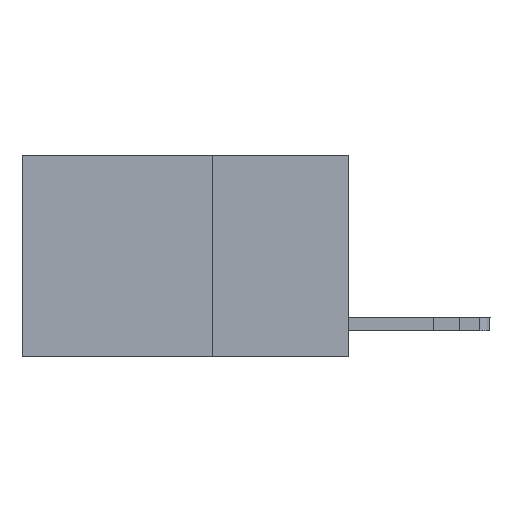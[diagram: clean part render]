
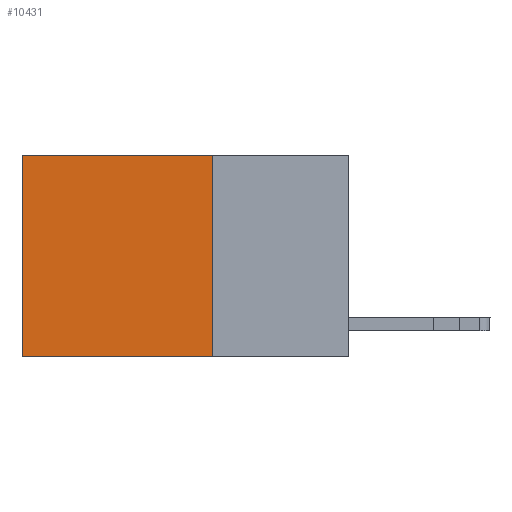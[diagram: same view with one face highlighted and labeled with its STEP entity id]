
A CAD part, left-side view. The second image highlights one B-rep face of the part: STEP entity #10431.
In plain terms, the highlighted planar face has unit normal (-1, 0, 0).
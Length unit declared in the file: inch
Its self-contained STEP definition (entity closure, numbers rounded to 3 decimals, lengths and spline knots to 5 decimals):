
#538 = PLANE ( 'NONE',  #15681 ) ;
#668 = VERTEX_POINT ( 'NONE', #9361 ) ;
#763 = ORIENTED_EDGE ( 'NONE', *, *, #8761, .F. ) ;
#1284 = EDGE_CURVE ( 'NONE', #5396, #668, #12461, .T. ) ;
#1404 = CARTESIAN_POINT ( 'NONE',  ( 0.2625, 0.6, -0.37 ) ) ;
#1964 = DIRECTION ( 'NONE',  ( 0., 0., -1. ) ) ;
#1974 = FACE_OUTER_BOUND ( 'NONE', #3654, .T. ) ;
#2413 = EDGE_CURVE ( 'NONE', #5396, #12620, #17888, .T. ) ;
#2499 = CARTESIAN_POINT ( 'NONE',  ( 0.2625, 0.25, 0. ) ) ;
#3436 = ORIENTED_EDGE ( 'NONE', *, *, #17680, .T. ) ;
#3442 = ORIENTED_EDGE ( 'NONE', *, *, #1284, .T. ) ;
#3654 = EDGE_LOOP ( 'NONE', ( #3436, #763, #15014, #3442 ) ) ;
#4782 = CARTESIAN_POINT ( 'NONE',  ( 0.2625, 0.6, 0. ) ) ;
#4869 = CARTESIAN_POINT ( 'NONE',  ( 0.2625, 0.25, 0. ) ) ;
#5059 = CARTESIAN_POINT ( 'NONE',  ( 0.2625, 0.25, -0.37 ) ) ;
#5396 = VERTEX_POINT ( 'NONE', #4869 ) ;
#6296 = DIRECTION ( 'NONE',  ( 1., 0., 0. ) ) ;
#7435 = VECTOR ( 'NONE', #1964, 39.37008 ) ;
#8305 = DIRECTION ( 'NONE',  ( 0., 1., 0. ) ) ;
#8761 = EDGE_CURVE ( 'NONE', #12620, #15531, #17094, .T. ) ;
#8991 = DIRECTION ( 'NONE',  ( 0., 0., -1. ) ) ;
#9052 = VECTOR ( 'NONE', #8305, 39.37008 ) ;
#9302 = VECTOR ( 'NONE', #12156, 39.37008 ) ;
#9361 = CARTESIAN_POINT ( 'NONE',  ( 0.2625, 0.6, 0. ) ) ;
#9695 = CARTESIAN_POINT ( 'NONE',  ( 0.2625, 0.25, -0.37 ) ) ;
#10421 = CARTESIAN_POINT ( 'NONE',  ( 0.2625, 0.25, 0. ) ) ;
#10431 = ADVANCED_FACE ( 'NONE', ( #1974 ), #538, .F. ) ;
#12156 = DIRECTION ( 'NONE',  ( 0., 1., 0. ) ) ;
#12461 = LINE ( 'NONE', #2499, #9302 ) ;
#12620 = VERTEX_POINT ( 'NONE', #5059 ) ;
#13477 = VECTOR ( 'NONE', #8991, 39.37008 ) ;
#15014 = ORIENTED_EDGE ( 'NONE', *, *, #2413, .F. ) ;
#15093 = LINE ( 'NONE', #4782, #7435 ) ;
#15531 = VERTEX_POINT ( 'NONE', #1404 ) ;
#15681 = AXIS2_PLACEMENT_3D ( 'NONE', #10421, #6296, #15832 ) ;
#15832 = DIRECTION ( 'NONE',  ( 0., 0., -1. ) ) ;
#17086 = CARTESIAN_POINT ( 'NONE',  ( 0.2625, 0.25, 0. ) ) ;
#17094 = LINE ( 'NONE', #9695, #9052 ) ;
#17680 = EDGE_CURVE ( 'NONE', #668, #15531, #15093, .T. ) ;
#17888 = LINE ( 'NONE', #17086, #13477 ) ;
